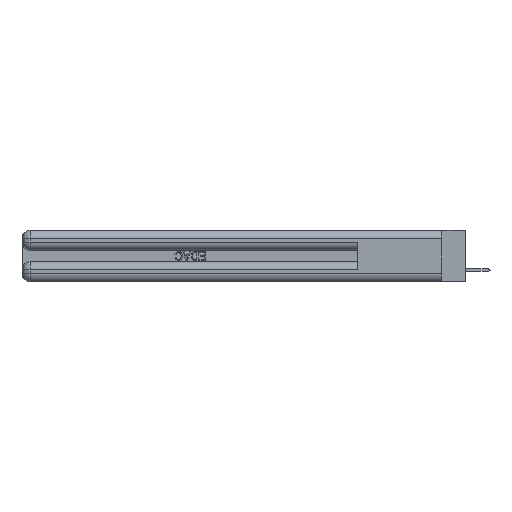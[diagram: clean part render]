
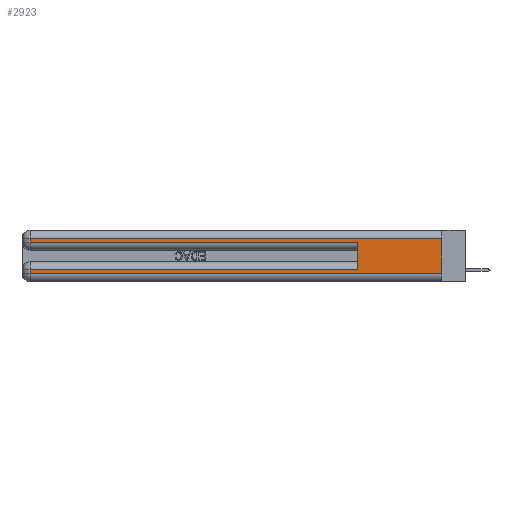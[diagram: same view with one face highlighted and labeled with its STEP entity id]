
A CAD part, left-side view. The second image highlights one B-rep face of the part: STEP entity #2923.
In plain terms, the highlighted planar face has unit normal (-1, 0, 0).
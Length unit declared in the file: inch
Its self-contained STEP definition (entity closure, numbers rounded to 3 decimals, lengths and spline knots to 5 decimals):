
#1854 = DIRECTION ( 'NONE',  ( 0., 1., 0. ) ) ;
#2606 = VECTOR ( 'NONE', #6776, 39.37008 ) ;
#2923 = ADVANCED_FACE ( 'NONE', ( #8592 ), #22585, .F. ) ;
#3032 = DIRECTION ( 'NONE',  ( 0., 0., -1. ) ) ;
#3052 = LINE ( 'NONE', #24860, #4007 ) ;
#3398 = CARTESIAN_POINT ( 'NONE',  ( 0., 2.94, 0.085 ) ) ;
#3620 = CARTESIAN_POINT ( 'NONE',  ( 0., 0., 0.285 ) ) ;
#3728 = CARTESIAN_POINT ( 'NONE',  ( 0., 2.94, 0.37 ) ) ;
#4007 = VECTOR ( 'NONE', #6001, 39.37008 ) ;
#4050 = CARTESIAN_POINT ( 'NONE',  ( 0., 0., 0.31 ) ) ;
#4828 = AXIS2_PLACEMENT_3D ( 'NONE', #10099, #35541, #19980 ) ;
#5468 = CARTESIAN_POINT ( 'NONE',  ( 0., 0., 0.06 ) ) ;
#6001 = DIRECTION ( 'NONE',  ( 0., 0., 1. ) ) ;
#6406 = EDGE_CURVE ( 'NONE', #36736, #30938, #32535, .T. ) ;
#6561 = EDGE_CURVE ( 'NONE', #6948, #35864, #3052, .T. ) ;
#6776 = DIRECTION ( 'NONE',  ( 0., -1., 0. ) ) ;
#6948 = VERTEX_POINT ( 'NONE', #17117 ) ;
#8592 = FACE_OUTER_BOUND ( 'NONE', #27732, .T. ) ;
#8755 = ORIENTED_EDGE ( 'NONE', *, *, #9541, .T. ) ;
#8885 = VECTOR ( 'NONE', #35310, 39.37008 ) ;
#9541 = EDGE_CURVE ( 'NONE', #29185, #35864, #15894, .T. ) ;
#10099 = CARTESIAN_POINT ( 'NONE',  ( 0., 0., 0.37 ) ) ;
#11187 = ORIENTED_EDGE ( 'NONE', *, *, #33285, .T. ) ;
#11880 = LINE ( 'NONE', #28991, #8885 ) ;
#12927 = ORIENTED_EDGE ( 'NONE', *, *, #29696, .F. ) ;
#13031 = LINE ( 'NONE', #39290, #32213 ) ;
#13597 = DIRECTION ( 'NONE',  ( 0., 0., -1. ) ) ;
#14492 = EDGE_CURVE ( 'NONE', #30938, #29185, #18682, .T. ) ;
#14892 = CARTESIAN_POINT ( 'NONE',  ( 0., 2.94, 0.31 ) ) ;
#15371 = VECTOR ( 'NONE', #28548, 39.37008 ) ;
#15591 = LINE ( 'NONE', #18145, #22925 ) ;
#15894 = LINE ( 'NONE', #3620, #2606 ) ;
#16096 = ORIENTED_EDGE ( 'NONE', *, *, #6406, .T. ) ;
#16579 = CARTESIAN_POINT ( 'NONE',  ( 0., 0., 0.31 ) ) ;
#17117 = CARTESIAN_POINT ( 'NONE',  ( 0., 0.6, 0.085 ) ) ;
#17558 = VECTOR ( 'NONE', #1854, 39.37008 ) ;
#18145 = CARTESIAN_POINT ( 'NONE',  ( 0., 2.94, 0.37 ) ) ;
#18682 = LINE ( 'NONE', #3728, #24178 ) ;
#18848 = VERTEX_POINT ( 'NONE', #3398 ) ;
#18975 = LINE ( 'NONE', #26464, #17558 ) ;
#19980 = DIRECTION ( 'NONE',  ( 0., 0., -1. ) ) ;
#20103 = ORIENTED_EDGE ( 'NONE', *, *, #37180, .T. ) ;
#22585 = PLANE ( 'NONE',  #4828 ) ;
#22925 = VECTOR ( 'NONE', #3032, 39.37008 ) ;
#24178 = VECTOR ( 'NONE', #27112, 39.37008 ) ;
#24860 = CARTESIAN_POINT ( 'NONE',  ( 0., 0.6, 0.145 ) ) ;
#26464 = CARTESIAN_POINT ( 'NONE',  ( 0., 0., 0.085 ) ) ;
#27112 = DIRECTION ( 'NONE',  ( 0., 0., -1. ) ) ;
#27732 = EDGE_LOOP ( 'NONE', ( #12927, #16096, #39080, #8755, #31501, #37582, #11187, #20103 ) ) ;
#28453 = EDGE_CURVE ( 'NONE', #6948, #18848, #18975, .T. ) ;
#28548 = DIRECTION ( 'NONE',  ( 0., 1., 0. ) ) ;
#28991 = CARTESIAN_POINT ( 'NONE',  ( 0., 0., 0.06 ) ) ;
#29185 = VERTEX_POINT ( 'NONE', #39616 ) ;
#29696 = EDGE_CURVE ( 'NONE', #36736, #36551, #13031, .T. ) ;
#30938 = VERTEX_POINT ( 'NONE', #14892 ) ;
#31501 = ORIENTED_EDGE ( 'NONE', *, *, #6561, .F. ) ;
#32213 = VECTOR ( 'NONE', #13597, 39.37008 ) ;
#32535 = LINE ( 'NONE', #4050, #15371 ) ;
#33285 = EDGE_CURVE ( 'NONE', #18848, #37533, #15591, .T. ) ;
#33785 = CARTESIAN_POINT ( 'NONE',  ( 0., 2.94, 0.06 ) ) ;
#35310 = DIRECTION ( 'NONE',  ( 0., -1., 0. ) ) ;
#35541 = DIRECTION ( 'NONE',  ( 1., 0., 0. ) ) ;
#35864 = VERTEX_POINT ( 'NONE', #36735 ) ;
#36551 = VERTEX_POINT ( 'NONE', #5468 ) ;
#36735 = CARTESIAN_POINT ( 'NONE',  ( 0., 0.6, 0.285 ) ) ;
#36736 = VERTEX_POINT ( 'NONE', #16579 ) ;
#37180 = EDGE_CURVE ( 'NONE', #37533, #36551, #11880, .T. ) ;
#37533 = VERTEX_POINT ( 'NONE', #33785 ) ;
#37582 = ORIENTED_EDGE ( 'NONE', *, *, #28453, .T. ) ;
#39080 = ORIENTED_EDGE ( 'NONE', *, *, #14492, .T. ) ;
#39290 = CARTESIAN_POINT ( 'NONE',  ( 0., 0., 0.37 ) ) ;
#39616 = CARTESIAN_POINT ( 'NONE',  ( 0., 2.94, 0.285 ) ) ;
